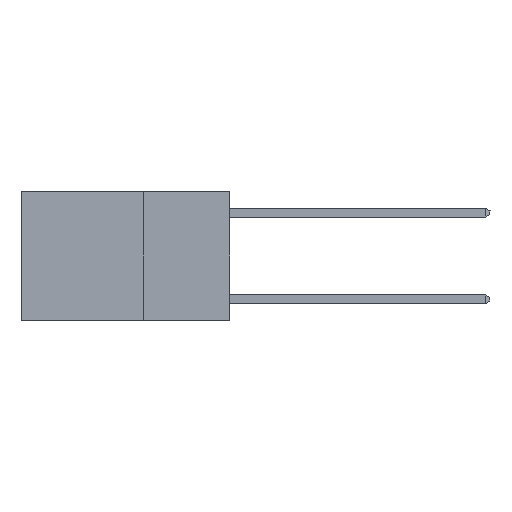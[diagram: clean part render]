
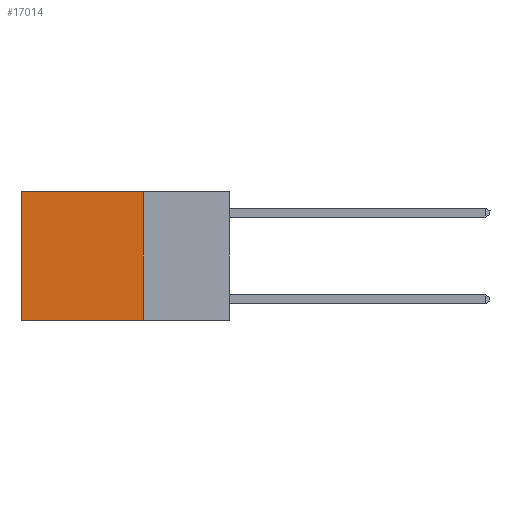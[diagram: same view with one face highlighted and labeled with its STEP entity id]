
A CAD part, left-side view. The second image highlights one B-rep face of the part: STEP entity #17014.
In plain terms, the highlighted planar face has unit normal (-1, 0, 0).
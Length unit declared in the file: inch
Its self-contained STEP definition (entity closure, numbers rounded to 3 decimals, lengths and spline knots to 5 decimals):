
#364 = ORIENTED_EDGE ( 'NONE', *, *, #7690, .F. ) ;
#495 = DIRECTION ( 'NONE',  ( 1., 0., 0. ) ) ;
#520 = EDGE_CURVE ( 'NONE', #10808, #17319, #16398, .T. ) ;
#3885 = DIRECTION ( 'NONE',  ( 0., 1., 0. ) ) ;
#4236 = LINE ( 'NONE', #4559, #14718 ) ;
#4559 = CARTESIAN_POINT ( 'NONE',  ( 0.2625, 0.6, 0. ) ) ;
#4666 = CARTESIAN_POINT ( 'NONE',  ( 0.2625, 0.25, 0. ) ) ;
#5941 = DIRECTION ( 'NONE',  ( 0., 0., -1. ) ) ;
#6594 = CARTESIAN_POINT ( 'NONE',  ( 0.2625, 0.25, -0.37 ) ) ;
#7544 = CARTESIAN_POINT ( 'NONE',  ( 0.2625, 0.25, 0. ) ) ;
#7690 = EDGE_CURVE ( 'NONE', #14236, #16836, #10458, .T. ) ;
#7729 = ORIENTED_EDGE ( 'NONE', *, *, #520, .T. ) ;
#9755 = VECTOR ( 'NONE', #14432, 39.37008 ) ;
#9935 = EDGE_LOOP ( 'NONE', ( #17086, #364, #13409, #7729 ) ) ;
#10201 = DIRECTION ( 'NONE',  ( 0., 0., -1. ) ) ;
#10458 = LINE ( 'NONE', #6594, #17108 ) ;
#10808 = VERTEX_POINT ( 'NONE', #7544 ) ;
#10901 = AXIS2_PLACEMENT_3D ( 'NONE', #4666, #495, #10201 ) ;
#12055 = EDGE_CURVE ( 'NONE', #10808, #14236, #12943, .T. ) ;
#12172 = DIRECTION ( 'NONE',  ( 0., 1., 0. ) ) ;
#12516 = CARTESIAN_POINT ( 'NONE',  ( 0.2625, 0.6, -0.37 ) ) ;
#12861 = VECTOR ( 'NONE', #12172, 39.37008 ) ;
#12943 = LINE ( 'NONE', #13067, #9755 ) ;
#13067 = CARTESIAN_POINT ( 'NONE',  ( 0.2625, 0.25, 0. ) ) ;
#13409 = ORIENTED_EDGE ( 'NONE', *, *, #12055, .F. ) ;
#13612 = CARTESIAN_POINT ( 'NONE',  ( 0.2625, 0.25, 0. ) ) ;
#13650 = FACE_OUTER_BOUND ( 'NONE', #9935, .T. ) ;
#14236 = VERTEX_POINT ( 'NONE', #14957 ) ;
#14432 = DIRECTION ( 'NONE',  ( 0., 0., -1. ) ) ;
#14718 = VECTOR ( 'NONE', #5941, 39.37008 ) ;
#14957 = CARTESIAN_POINT ( 'NONE',  ( 0.2625, 0.25, -0.37 ) ) ;
#16337 = EDGE_CURVE ( 'NONE', #17319, #16836, #4236, .T. ) ;
#16398 = LINE ( 'NONE', #13612, #12861 ) ;
#16836 = VERTEX_POINT ( 'NONE', #12516 ) ;
#16841 = PLANE ( 'NONE',  #10901 ) ;
#17014 = ADVANCED_FACE ( 'NONE', ( #13650 ), #16841, .F. ) ;
#17086 = ORIENTED_EDGE ( 'NONE', *, *, #16337, .T. ) ;
#17108 = VECTOR ( 'NONE', #3885, 39.37008 ) ;
#17319 = VERTEX_POINT ( 'NONE', #17331 ) ;
#17331 = CARTESIAN_POINT ( 'NONE',  ( 0.2625, 0.6, 0. ) ) ;
